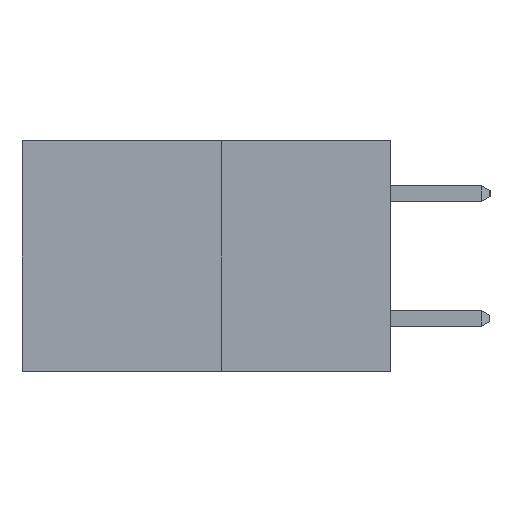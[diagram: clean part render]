
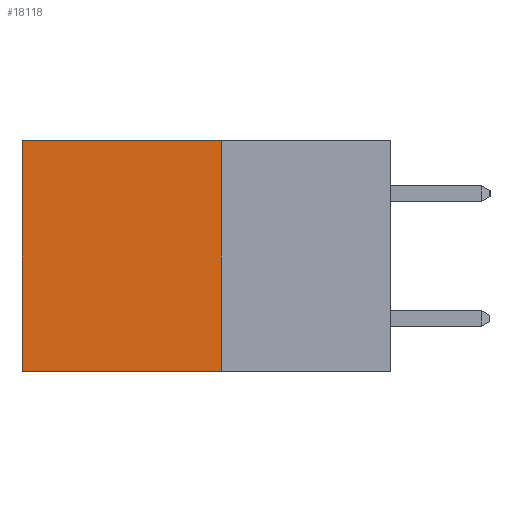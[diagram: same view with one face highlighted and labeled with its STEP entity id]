
A CAD part, left-side view. The second image highlights one B-rep face of the part: STEP entity #18118.
In plain terms, the highlighted planar face has unit normal (-1, 0, 0).
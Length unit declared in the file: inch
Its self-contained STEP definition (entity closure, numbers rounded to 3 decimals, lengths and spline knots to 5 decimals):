
#279 = EDGE_CURVE ( 'NONE', #4765, #8934, #16820, .T. ) ;
#1268 = DIRECTION ( 'NONE',  ( 0., 1., 0. ) ) ;
#1465 = AXIS2_PLACEMENT_3D ( 'NONE', #19601, #3412, #16023 ) ;
#1812 = DIRECTION ( 'NONE',  ( 0., 1., 0. ) ) ;
#3412 = DIRECTION ( 'NONE',  ( 1., 0., 0. ) ) ;
#4048 = VECTOR ( 'NONE', #14012, 39.37008 ) ;
#4765 = VERTEX_POINT ( 'NONE', #18629 ) ;
#5354 = VECTOR ( 'NONE', #1812, 39.37008 ) ;
#6294 = EDGE_CURVE ( 'NONE', #22676, #13174, #22059, .T. ) ;
#6818 = DIRECTION ( 'NONE',  ( 0., 0., -1. ) ) ;
#7168 = CARTESIAN_POINT ( 'NONE',  ( 0.277, 0.59, 0. ) ) ;
#7305 = CARTESIAN_POINT ( 'NONE',  ( 0.277, 0.27, 0. ) ) ;
#7321 = VECTOR ( 'NONE', #6818, 39.37008 ) ;
#8934 = VERTEX_POINT ( 'NONE', #12916 ) ;
#9526 = CARTESIAN_POINT ( 'NONE',  ( 0.277, 0.59, -0.37 ) ) ;
#9804 = EDGE_LOOP ( 'NONE', ( #12556, #16765, #21212, #20831 ) ) ;
#9950 = LINE ( 'NONE', #22850, #18926 ) ;
#10656 = PLANE ( 'NONE',  #1465 ) ;
#11413 = FACE_OUTER_BOUND ( 'NONE', #9804, .T. ) ;
#12556 = ORIENTED_EDGE ( 'NONE', *, *, #6294, .T. ) ;
#12916 = CARTESIAN_POINT ( 'NONE',  ( 0.277, 0.27, -0.37 ) ) ;
#13174 = VERTEX_POINT ( 'NONE', #21567 ) ;
#14012 = DIRECTION ( 'NONE',  ( 0., 0., -1. ) ) ;
#14312 = LINE ( 'NONE', #7305, #5354 ) ;
#15284 = EDGE_CURVE ( 'NONE', #4765, #22676, #14312, .T. ) ;
#16023 = DIRECTION ( 'NONE',  ( 0., 0., -1. ) ) ;
#16765 = ORIENTED_EDGE ( 'NONE', *, *, #20202, .F. ) ;
#16820 = LINE ( 'NONE', #19658, #7321 ) ;
#18118 = ADVANCED_FACE ( 'NONE', ( #11413 ), #10656, .F. ) ;
#18629 = CARTESIAN_POINT ( 'NONE',  ( 0.277, 0.27, 0. ) ) ;
#18926 = VECTOR ( 'NONE', #1268, 39.37008 ) ;
#19601 = CARTESIAN_POINT ( 'NONE',  ( 0.277, 0.27, -0.37 ) ) ;
#19658 = CARTESIAN_POINT ( 'NONE',  ( 0.277, 0.27, -0.37 ) ) ;
#20202 = EDGE_CURVE ( 'NONE', #8934, #13174, #9950, .T. ) ;
#20831 = ORIENTED_EDGE ( 'NONE', *, *, #15284, .T. ) ;
#21212 = ORIENTED_EDGE ( 'NONE', *, *, #279, .F. ) ;
#21567 = CARTESIAN_POINT ( 'NONE',  ( 0.277, 0.59, -0.37 ) ) ;
#22059 = LINE ( 'NONE', #9526, #4048 ) ;
#22676 = VERTEX_POINT ( 'NONE', #7168 ) ;
#22850 = CARTESIAN_POINT ( 'NONE',  ( 0.277, 0.27, -0.37 ) ) ;
